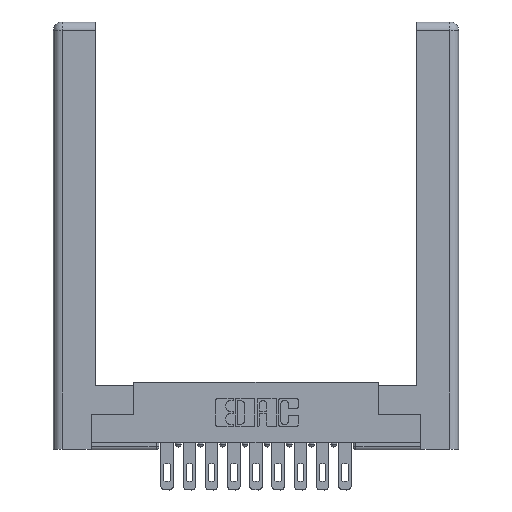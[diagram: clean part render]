
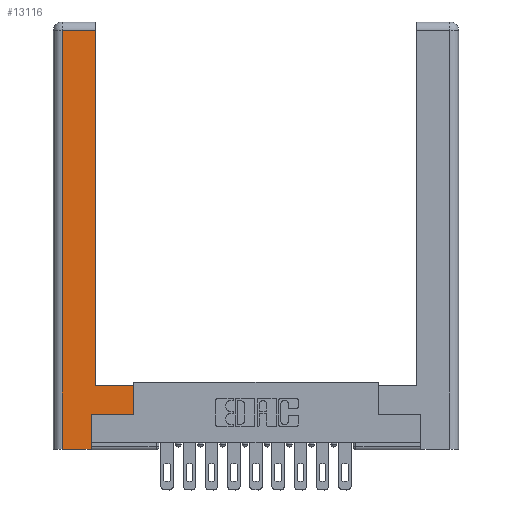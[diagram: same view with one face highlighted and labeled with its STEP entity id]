
A CAD part, top view. The second image highlights one B-rep face of the part: STEP entity #13116.
In plain terms, the highlighted planar face has unit normal (0, 0, 1).
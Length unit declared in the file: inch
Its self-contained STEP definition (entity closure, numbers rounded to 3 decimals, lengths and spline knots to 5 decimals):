
#62 = DIRECTION ( 'NONE',  ( 1., 0., 0. ) ) ;
#132 = ORIENTED_EDGE ( 'NONE', *, *, #8493, .T. ) ;
#388 = VERTEX_POINT ( 'NONE', #1954 ) ;
#490 = VERTEX_POINT ( 'NONE', #3359 ) ;
#719 = EDGE_CURVE ( 'NONE', #388, #1090, #7723, .T. ) ;
#782 = VECTOR ( 'NONE', #4639, 39.37008 ) ;
#1090 = VERTEX_POINT ( 'NONE', #9701 ) ;
#1174 = LINE ( 'NONE', #12543, #12406 ) ;
#1353 = ORIENTED_EDGE ( 'NONE', *, *, #10653, .T. ) ;
#1441 = VECTOR ( 'NONE', #7898, 39.37008 ) ;
#1490 = VECTOR ( 'NONE', #13775, 39.37008 ) ;
#1517 = EDGE_CURVE ( 'NONE', #1090, #6650, #2636, .T. ) ;
#1664 = CARTESIAN_POINT ( 'NONE',  ( 0.0615, 2.94, 0. ) ) ;
#1954 = CARTESIAN_POINT ( 'NONE',  ( 0.295, 0.45, 0. ) ) ;
#2149 = VECTOR ( 'NONE', #6921, 39.37008 ) ;
#2178 = CARTESIAN_POINT ( 'NONE',  ( 0.565, 0.245, 0. ) ) ;
#2615 = CARTESIAN_POINT ( 'NONE',  ( 0.265, 0., 0. ) ) ;
#2636 = LINE ( 'NONE', #1664, #9202 ) ;
#2691 = PLANE ( 'NONE',  #8612 ) ;
#3050 = LINE ( 'NONE', #4226, #1441 ) ;
#3345 = CARTESIAN_POINT ( 'NONE',  ( 0.265, 0., 0. ) ) ;
#3359 = CARTESIAN_POINT ( 'NONE',  ( 0.0615, 0., 0. ) ) ;
#3368 = VERTEX_POINT ( 'NONE', #3345 ) ;
#3409 = CARTESIAN_POINT ( 'NONE',  ( 0.565, 0.245, 0. ) ) ;
#3572 = CARTESIAN_POINT ( 'NONE',  ( 0., 0., 0. ) ) ;
#3821 = CARTESIAN_POINT ( 'NONE',  ( 0.0615, 0., 0. ) ) ;
#3937 = CARTESIAN_POINT ( 'NONE',  ( 0.0615, 2.94, 0. ) ) ;
#4184 = CARTESIAN_POINT ( 'NONE',  ( 0.565, 0.45, 0. ) ) ;
#4226 = CARTESIAN_POINT ( 'NONE',  ( 0.565, 0.45, 0. ) ) ;
#4599 = CARTESIAN_POINT ( 'NONE',  ( 0.295, 0.45, 0. ) ) ;
#4639 = DIRECTION ( 'NONE',  ( 0., -1., 0. ) ) ;
#4884 = VERTEX_POINT ( 'NONE', #2178 ) ;
#4918 = FACE_OUTER_BOUND ( 'NONE', #4923, .T. ) ;
#4923 = EDGE_LOOP ( 'NONE', ( #9366, #8446, #132, #6477, #7758, #12704, #1353, #13531 ) ) ;
#5633 = CARTESIAN_POINT ( 'NONE',  ( 0.295, 3., 0. ) ) ;
#6477 = ORIENTED_EDGE ( 'NONE', *, *, #13109, .T. ) ;
#6650 = VERTEX_POINT ( 'NONE', #3937 ) ;
#6918 = LINE ( 'NONE', #3409, #12977 ) ;
#6921 = DIRECTION ( 'NONE',  ( -1., 0., 0. ) ) ;
#7150 = DIRECTION ( 'NONE',  ( 0., 0., -1. ) ) ;
#7181 = LINE ( 'NONE', #3821, #782 ) ;
#7388 = DIRECTION ( 'NONE',  ( -1., 0., 0. ) ) ;
#7399 = EDGE_CURVE ( 'NONE', #3368, #9187, #1174, .T. ) ;
#7723 = LINE ( 'NONE', #5633, #9185 ) ;
#7758 = ORIENTED_EDGE ( 'NONE', *, *, #7399, .T. ) ;
#7898 = DIRECTION ( 'NONE',  ( 0., 1., 0. ) ) ;
#8446 = ORIENTED_EDGE ( 'NONE', *, *, #1517, .T. ) ;
#8493 = EDGE_CURVE ( 'NONE', #6650, #490, #7181, .T. ) ;
#8612 = AXIS2_PLACEMENT_3D ( 'NONE', #3572, #7150, #11693 ) ;
#9185 = VECTOR ( 'NONE', #12085, 39.37008 ) ;
#9187 = VERTEX_POINT ( 'NONE', #13993 ) ;
#9202 = VECTOR ( 'NONE', #7388, 39.37008 ) ;
#9366 = ORIENTED_EDGE ( 'NONE', *, *, #719, .T. ) ;
#9422 = EDGE_CURVE ( 'NONE', #9187, #4884, #6918, .T. ) ;
#9701 = CARTESIAN_POINT ( 'NONE',  ( 0.295, 2.94, 0. ) ) ;
#10184 = LINE ( 'NONE', #4599, #2149 ) ;
#10243 = DIRECTION ( 'NONE',  ( 0., 1., 0. ) ) ;
#10653 = EDGE_CURVE ( 'NONE', #4884, #14049, #3050, .T. ) ;
#10847 = EDGE_CURVE ( 'NONE', #14049, #388, #10184, .T. ) ;
#11693 = DIRECTION ( 'NONE',  ( -1., 0., 0. ) ) ;
#12085 = DIRECTION ( 'NONE',  ( 0., 1., 0. ) ) ;
#12406 = VECTOR ( 'NONE', #10243, 39.37008 ) ;
#12543 = CARTESIAN_POINT ( 'NONE',  ( 0.265, 0.245, 0. ) ) ;
#12704 = ORIENTED_EDGE ( 'NONE', *, *, #9422, .T. ) ;
#12798 = LINE ( 'NONE', #2615, #1490 ) ;
#12977 = VECTOR ( 'NONE', #62, 39.37008 ) ;
#13109 = EDGE_CURVE ( 'NONE', #490, #3368, #12798, .T. ) ;
#13116 = ADVANCED_FACE ( 'NONE', ( #4918 ), #2691, .F. ) ;
#13531 = ORIENTED_EDGE ( 'NONE', *, *, #10847, .T. ) ;
#13775 = DIRECTION ( 'NONE',  ( 1., 0., 0. ) ) ;
#13993 = CARTESIAN_POINT ( 'NONE',  ( 0.265, 0.245, 0. ) ) ;
#14049 = VERTEX_POINT ( 'NONE', #4184 ) ;
